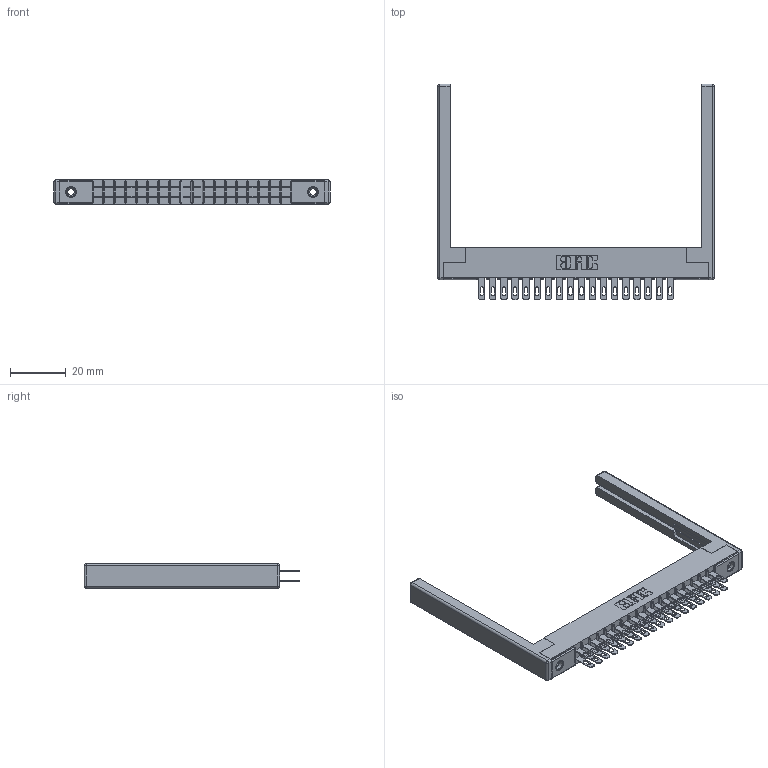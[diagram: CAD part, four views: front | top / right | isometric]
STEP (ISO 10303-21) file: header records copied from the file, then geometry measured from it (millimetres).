
FILE_DESCRIPTION (( 'STEP AP203' ), '1' );
FILE_NAME ('315-036-500-268.STEP', '2019-09-10T16:06:15', ( '' ), ( '' ), 'SwSTEP 2.0', 'SolidWorks 2016', '' );
FILE_SCHEMA (( 'CONFIG_CONTROL_DESIGN' ));
Length unit declared in the file: inch
Products named in the file (5): 315-036-500-268; 345-250-001_345-250-001-102; 305-290-001_500; 307-220-068; 305 Part_.156 Dia
Assembly tree (41 placements, depth 2):
  315-036-500-268
    305 Part_.156 Dia
    305-290-001_500  x36
    345-250-001_345-250-001-102  x2
    307-220-068  x2
Bounding box: 98.76 x 77.14 x 8.71 mm (x, y, z)
Volume: 10888.2 mm3; surface area: 16344.4 mm2
Topology: 41 solids, 41 shells, 2070 faces, 5872 edges, 3796 vertices
Faces by surface type: plane 1164, cylinder 810, sphere 80, cone 12, torus 4
Entity records: 25192 total; most frequent: CARTESIAN_POINT 4141, ORIENTED_EDGE 4098, DIRECTION 4047, EDGE_CURVE 2049, LINE 1619, VECTOR 1619, VERTEX_POINT 1308, AXIS2_PLACEMENT_3D 1214
